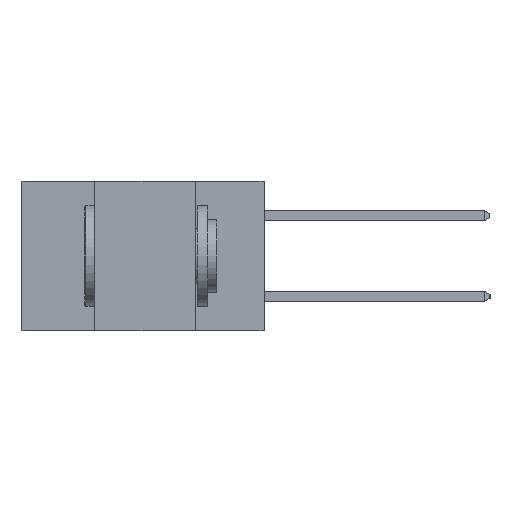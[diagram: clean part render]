
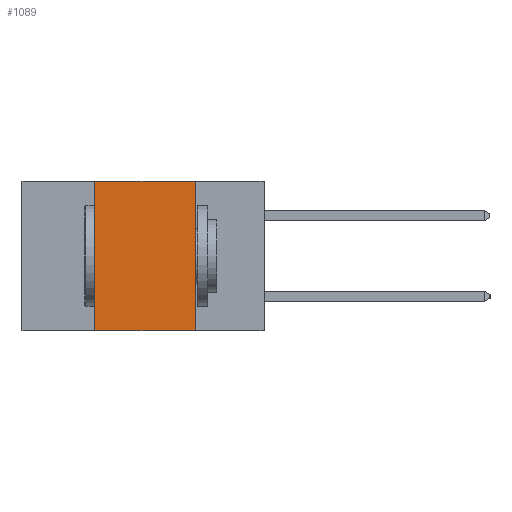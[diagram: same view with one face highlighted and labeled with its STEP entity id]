
A CAD part, left-side view. The second image highlights one B-rep face of the part: STEP entity #1089.
In plain terms, the highlighted planar face has unit normal (-1, 0, 0).
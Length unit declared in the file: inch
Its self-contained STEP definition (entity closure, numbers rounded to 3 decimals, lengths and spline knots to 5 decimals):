
#939 = ORIENTED_EDGE ( 'NONE', *, *, #6578, .F. ) ;
#1089 = ADVANCED_FACE ( 'NONE', ( #11785 ), #8293, .F. ) ;
#1184 = CARTESIAN_POINT ( 'NONE',  ( 0., 0.6, 0. ) ) ;
#1583 = VERTEX_POINT ( 'NONE', #9225 ) ;
#1614 = CARTESIAN_POINT ( 'NONE',  ( 0., 0.6, -0.37 ) ) ;
#2130 = LINE ( 'NONE', #13499, #12000 ) ;
#2214 = EDGE_CURVE ( 'NONE', #14078, #1583, #14937, .T. ) ;
#3874 = CARTESIAN_POINT ( 'NONE',  ( 0., 0.6, 0. ) ) ;
#3974 = DIRECTION ( 'NONE',  ( 0., -1., 0. ) ) ;
#4736 = VECTOR ( 'NONE', #3974, 39.37008 ) ;
#5225 = DIRECTION ( 'NONE',  ( 0., 0., -1. ) ) ;
#5565 = CARTESIAN_POINT ( 'NONE',  ( 0., 0.17, -0.37 ) ) ;
#6578 = EDGE_CURVE ( 'NONE', #1583, #10457, #2130, .T. ) ;
#6673 = VECTOR ( 'NONE', #7467, 39.37008 ) ;
#6809 = CARTESIAN_POINT ( 'NONE',  ( 0., 0.42, 0. ) ) ;
#7303 = ORIENTED_EDGE ( 'NONE', *, *, #2214, .F. ) ;
#7467 = DIRECTION ( 'NONE',  ( 0., 0., 1. ) ) ;
#8214 = EDGE_LOOP ( 'NONE', ( #939, #7303, #9271, #10038 ) ) ;
#8293 = PLANE ( 'NONE',  #13937 ) ;
#8509 = DIRECTION ( 'NONE',  ( 1., 0., 0. ) ) ;
#9125 = DIRECTION ( 'NONE',  ( 0., 0., -1. ) ) ;
#9225 = CARTESIAN_POINT ( 'NONE',  ( 0., 0.17, 0. ) ) ;
#9271 = ORIENTED_EDGE ( 'NONE', *, *, #16237, .F. ) ;
#9673 = VECTOR ( 'NONE', #10603, 39.37008 ) ;
#10038 = ORIENTED_EDGE ( 'NONE', *, *, #15411, .T. ) ;
#10457 = VERTEX_POINT ( 'NONE', #5565 ) ;
#10603 = DIRECTION ( 'NONE',  ( 0., -1., 0. ) ) ;
#10828 = VERTEX_POINT ( 'NONE', #13575 ) ;
#11785 = FACE_OUTER_BOUND ( 'NONE', #8214, .T. ) ;
#12000 = VECTOR ( 'NONE', #9125, 39.37008 ) ;
#13089 = LINE ( 'NONE', #1614, #9673 ) ;
#13451 = LINE ( 'NONE', #16281, #6673 ) ;
#13499 = CARTESIAN_POINT ( 'NONE',  ( 0., 0.17, -0.37 ) ) ;
#13575 = CARTESIAN_POINT ( 'NONE',  ( 0., 0.42, -0.37 ) ) ;
#13937 = AXIS2_PLACEMENT_3D ( 'NONE', #1184, #8509, #5225 ) ;
#14078 = VERTEX_POINT ( 'NONE', #6809 ) ;
#14937 = LINE ( 'NONE', #3874, #4736 ) ;
#15411 = EDGE_CURVE ( 'NONE', #10828, #10457, #13089, .T. ) ;
#16237 = EDGE_CURVE ( 'NONE', #10828, #14078, #13451, .T. ) ;
#16281 = CARTESIAN_POINT ( 'NONE',  ( 0., 0.42, -0.37 ) ) ;
